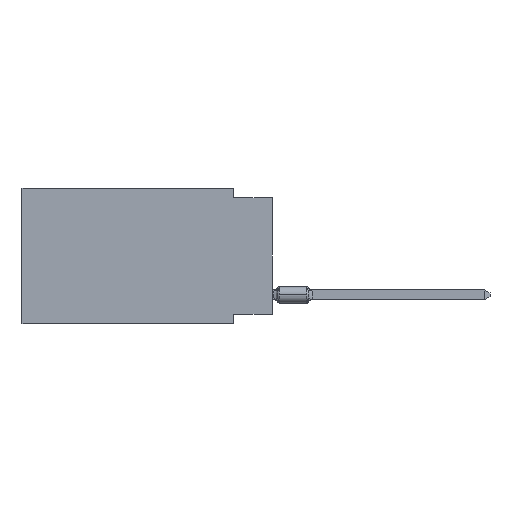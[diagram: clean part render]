
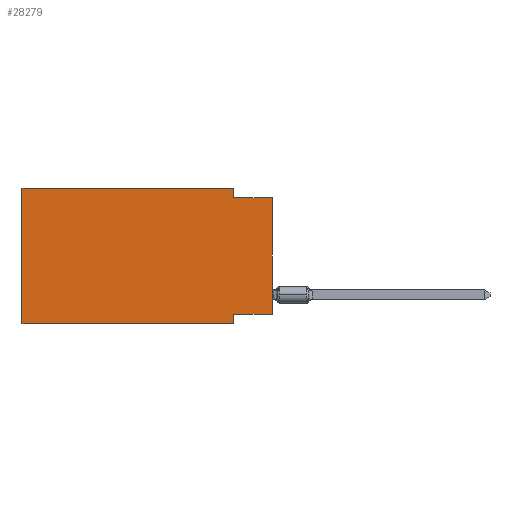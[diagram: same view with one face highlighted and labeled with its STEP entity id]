
A CAD part, left-side view. The second image highlights one B-rep face of the part: STEP entity #28279.
In plain terms, the highlighted planar face has unit normal (-1, 0, 0).
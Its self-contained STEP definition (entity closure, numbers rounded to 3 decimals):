
#432 = CARTESIAN_POINT ( 'NONE',  ( 0., 2.54, 0. ) ) ;
#490 = VECTOR ( 'NONE', #28585, 1000. ) ;
#662 = VERTEX_POINT ( 'NONE', #23988 ) ;
#818 = EDGE_CURVE ( 'NONE', #5943, #662, #22232, .T. ) ;
#1084 = VERTEX_POINT ( 'NONE', #3199 ) ;
#2328 = LINE ( 'NONE', #432, #9416 ) ;
#2789 = LINE ( 'NONE', #3231, #3543 ) ;
#3199 = CARTESIAN_POINT ( 'NONE',  ( 0., 2.54, 0. ) ) ;
#3231 = CARTESIAN_POINT ( 'NONE',  ( 0., 0., 0. ) ) ;
#3543 = VECTOR ( 'NONE', #12170, 1000. ) ;
#4093 = ORIENTED_EDGE ( 'NONE', *, *, #7993, .F. ) ;
#4649 = CARTESIAN_POINT ( 'NONE',  ( 0., 2.54, -0.635 ) ) ;
#4727 = EDGE_CURVE ( 'NONE', #1084, #9472, #2328, .T. ) ;
#5860 = VERTEX_POINT ( 'NONE', #26497 ) ;
#5921 = VERTEX_POINT ( 'NONE', #24595 ) ;
#5943 = VERTEX_POINT ( 'NONE', #24746 ) ;
#6046 = VECTOR ( 'NONE', #25001, 1000. ) ;
#6756 = ORIENTED_EDGE ( 'NONE', *, *, #8491, .T. ) ;
#6780 = ORIENTED_EDGE ( 'NONE', *, *, #13447, .F. ) ;
#7597 = CARTESIAN_POINT ( 'NONE',  ( 0., 16.383, 0. ) ) ;
#7736 = EDGE_CURVE ( 'NONE', #5943, #15633, #2789, .T. ) ;
#7767 = LINE ( 'NONE', #21372, #20849 ) ;
#7993 = EDGE_CURVE ( 'NONE', #662, #20818, #7767, .T. ) ;
#8491 = EDGE_CURVE ( 'NONE', #5860, #20818, #12820, .T. ) ;
#8696 = VECTOR ( 'NONE', #18554, 1000. ) ;
#9286 = PLANE ( 'NONE',  #10663 ) ;
#9416 = VECTOR ( 'NONE', #22664, 1000. ) ;
#9472 = VERTEX_POINT ( 'NONE', #4649 ) ;
#9939 = VECTOR ( 'NONE', #26426, 1000. ) ;
#10561 = CARTESIAN_POINT ( 'NONE',  ( 0., 2.54, -8.89 ) ) ;
#10663 = AXIS2_PLACEMENT_3D ( 'NONE', #26991, #20552, #28907 ) ;
#11492 = VECTOR ( 'NONE', #13774, 1000. ) ;
#12170 = DIRECTION ( 'NONE',  ( 0., 0., 1. ) ) ;
#12284 = LINE ( 'NONE', #7597, #8696 ) ;
#12820 = LINE ( 'NONE', #24384, #9939 ) ;
#12913 = CARTESIAN_POINT ( 'NONE',  ( 0., 16.383, 0. ) ) ;
#13328 = ORIENTED_EDGE ( 'NONE', *, *, #24618, .F. ) ;
#13447 = EDGE_CURVE ( 'NONE', #9472, #15633, #18447, .T. ) ;
#13774 = DIRECTION ( 'NONE',  ( 0., -1., 0. ) ) ;
#13921 = EDGE_CURVE ( 'NONE', #5860, #5921, #12284, .T. ) ;
#15084 = ORIENTED_EDGE ( 'NONE', *, *, #7736, .T. ) ;
#15633 = VERTEX_POINT ( 'NONE', #28742 ) ;
#16601 = ORIENTED_EDGE ( 'NONE', *, *, #4727, .F. ) ;
#17250 = DIRECTION ( 'NONE',  ( 0., 0., -1. ) ) ;
#17835 = ORIENTED_EDGE ( 'NONE', *, *, #13921, .F. ) ;
#18447 = LINE ( 'NONE', #24905, #11492 ) ;
#18554 = DIRECTION ( 'NONE',  ( 0., 0., 1. ) ) ;
#19202 = LINE ( 'NONE', #12913, #490 ) ;
#20552 = DIRECTION ( 'NONE',  ( 1., 0., 0. ) ) ;
#20818 = VERTEX_POINT ( 'NONE', #10561 ) ;
#20849 = VECTOR ( 'NONE', #17250, 1000. ) ;
#20978 = ORIENTED_EDGE ( 'NONE', *, *, #818, .F. ) ;
#21372 = CARTESIAN_POINT ( 'NONE',  ( 0., 2.54, -8.89 ) ) ;
#22232 = LINE ( 'NONE', #27200, #6046 ) ;
#22664 = DIRECTION ( 'NONE',  ( 0., 0., -1. ) ) ;
#23988 = CARTESIAN_POINT ( 'NONE',  ( 0., 2.54, -8.255 ) ) ;
#24384 = CARTESIAN_POINT ( 'NONE',  ( 0., 16.383, -8.89 ) ) ;
#24595 = CARTESIAN_POINT ( 'NONE',  ( 0., 16.383, 0. ) ) ;
#24618 = EDGE_CURVE ( 'NONE', #5921, #1084, #19202, .T. ) ;
#24650 = FACE_OUTER_BOUND ( 'NONE', #27655, .T. ) ;
#24746 = CARTESIAN_POINT ( 'NONE',  ( 0., 0., -8.255 ) ) ;
#24905 = CARTESIAN_POINT ( 'NONE',  ( 0., 0., -0.635 ) ) ;
#25001 = DIRECTION ( 'NONE',  ( 0., 1., 0. ) ) ;
#26426 = DIRECTION ( 'NONE',  ( 0., -1., 0. ) ) ;
#26497 = CARTESIAN_POINT ( 'NONE',  ( 0., 16.383, -8.89 ) ) ;
#26991 = CARTESIAN_POINT ( 'NONE',  ( 0., 16.383, 0. ) ) ;
#27200 = CARTESIAN_POINT ( 'NONE',  ( 0., 0., -8.255 ) ) ;
#27655 = EDGE_LOOP ( 'NONE', ( #15084, #6780, #16601, #13328, #17835, #6756, #4093, #20978 ) ) ;
#28279 = ADVANCED_FACE ( 'NONE', ( #24650 ), #9286, .F. ) ;
#28585 = DIRECTION ( 'NONE',  ( 0., -1., 0. ) ) ;
#28742 = CARTESIAN_POINT ( 'NONE',  ( 0., 0., -0.635 ) ) ;
#28907 = DIRECTION ( 'NONE',  ( 0., 0., -1. ) ) ;
